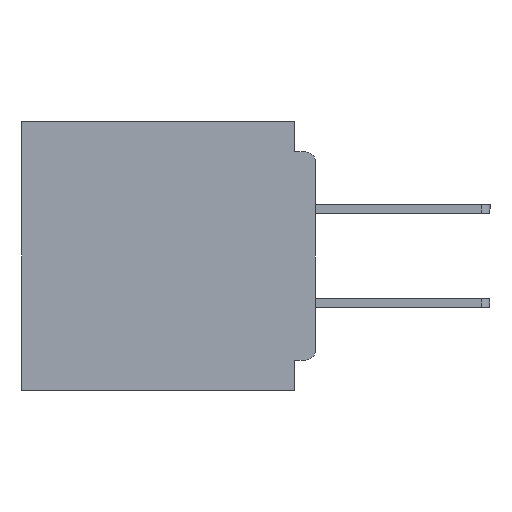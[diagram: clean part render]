
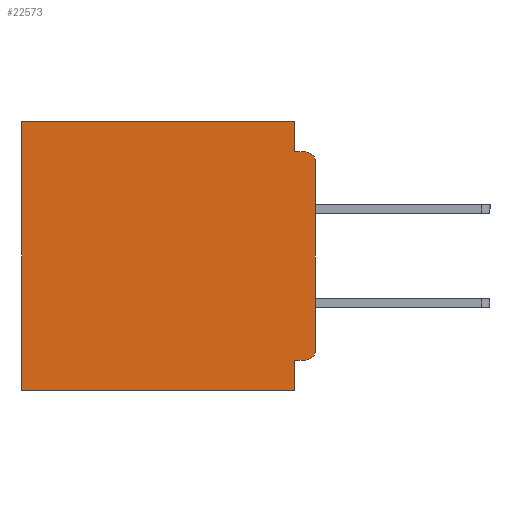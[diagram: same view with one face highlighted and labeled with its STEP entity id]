
A CAD part, left-side view. The second image highlights one B-rep face of the part: STEP entity #22573.
In plain terms, the highlighted planar face has unit normal (-1, 0, 0).
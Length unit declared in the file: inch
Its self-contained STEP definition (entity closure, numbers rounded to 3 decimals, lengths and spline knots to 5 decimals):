
#360 = CARTESIAN_POINT ( 'NONE',  ( 0.3, 0.031, -0.045 ) ) ;
#1058 = EDGE_CURVE ( 'NONE', #40323, #13940, #42511, .T. ) ;
#1134 = VECTOR ( 'NONE', #15272, 39.37008 ) ;
#2151 = AXIS2_PLACEMENT_3D ( 'NONE', #38801, #38703, #38646 ) ;
#2222 = LINE ( 'NONE', #35796, #1134 ) ;
#3002 = LINE ( 'NONE', #27524, #11056 ) ;
#3090 = PLANE ( 'NONE',  #3315 ) ;
#3315 = AXIS2_PLACEMENT_3D ( 'NONE', #33813, #13434, #37196 ) ;
#3655 = ORIENTED_EDGE ( 'NONE', *, *, #3857, .T. ) ;
#3857 = EDGE_CURVE ( 'NONE', #11465, #38300, #28055, .T. ) ;
#4116 = CARTESIAN_POINT ( 'NONE',  ( 0.3, 0., -0.34 ) ) ;
#4118 = ORIENTED_EDGE ( 'NONE', *, *, #21369, .F. ) ;
#5017 = EDGE_CURVE ( 'NONE', #40323, #13606, #28481, .T. ) ;
#5478 = ORIENTED_EDGE ( 'NONE', *, *, #30037, .T. ) ;
#6442 = VECTOR ( 'NONE', #20470, 39.37008 ) ;
#6855 = CARTESIAN_POINT ( 'NONE',  ( 0.3, 0.031, -0.355 ) ) ;
#6873 = ORIENTED_EDGE ( 'NONE', *, *, #43260, .F. ) ;
#7458 = DIRECTION ( 'NONE',  ( 0., 1., 0. ) ) ;
#8053 = VERTEX_POINT ( 'NONE', #24071 ) ;
#8957 = VECTOR ( 'NONE', #23183, 39.37008 ) ;
#9255 = ORIENTED_EDGE ( 'NONE', *, *, #5017, .T. ) ;
#10551 = DIRECTION ( 'NONE',  ( 0., 0., -1. ) ) ;
#10591 = EDGE_LOOP ( 'NONE', ( #35270, #9255, #6873, #4118, #3655, #15783, #39187, #33920, #41246, #5478 ) ) ;
#11056 = VECTOR ( 'NONE', #10551, 39.37008 ) ;
#11465 = VERTEX_POINT ( 'NONE', #25578 ) ;
#11623 = CARTESIAN_POINT ( 'NONE',  ( 0.3, 0., 0. ) ) ;
#12461 = DIRECTION ( 'NONE',  ( 0., 1., 0. ) ) ;
#13434 = DIRECTION ( 'NONE',  ( 1., 0., 0. ) ) ;
#13520 = VECTOR ( 'NONE', #39422, 39.37008 ) ;
#13606 = VERTEX_POINT ( 'NONE', #19066 ) ;
#13940 = VERTEX_POINT ( 'NONE', #4116 ) ;
#15272 = DIRECTION ( 'NONE',  ( 0., 0., -1. ) ) ;
#15783 = ORIENTED_EDGE ( 'NONE', *, *, #20322, .T. ) ;
#16253 = LINE ( 'NONE', #24460, #26403 ) ;
#16724 = CARTESIAN_POINT ( 'NONE',  ( 0.3, 0., -0.4 ) ) ;
#16883 = DIRECTION ( 'NONE',  ( 0., 1., 0. ) ) ;
#17685 = CARTESIAN_POINT ( 'NONE',  ( 0.3, 0.437, 0. ) ) ;
#18332 = CARTESIAN_POINT ( 'NONE',  ( 0.3, 0.015, -0.34 ) ) ;
#19066 = CARTESIAN_POINT ( 'NONE',  ( 0.3, 0.015, -0.045 ) ) ;
#19081 = CARTESIAN_POINT ( 'NONE',  ( 0.3, 0., -0.045 ) ) ;
#19359 = VERTEX_POINT ( 'NONE', #360 ) ;
#20322 = EDGE_CURVE ( 'NONE', #38300, #40238, #35038, .T. ) ;
#20384 = CIRCLE ( 'NONE', #27790, 0.015 ) ;
#20470 = DIRECTION ( 'NONE',  ( 0., 0., -1. ) ) ;
#21369 = EDGE_CURVE ( 'NONE', #11465, #19359, #3002, .T. ) ;
#21702 = CARTESIAN_POINT ( 'NONE',  ( 0.3, 0., -0.06 ) ) ;
#21775 = DIRECTION ( 'NONE',  ( 0., 0., -1. ) ) ;
#22573 = ADVANCED_FACE ( 'NONE', ( #36468 ), #3090, .F. ) ;
#22600 = EDGE_CURVE ( 'NONE', #24616, #40238, #16253, .T. ) ;
#22658 = CARTESIAN_POINT ( 'NONE',  ( 0.3, 0.031, -0.4 ) ) ;
#23183 = DIRECTION ( 'NONE',  ( 0., 0., -1. ) ) ;
#23650 = LINE ( 'NONE', #19081, #13520 ) ;
#23916 = EDGE_CURVE ( 'NONE', #32788, #24616, #2222, .T. ) ;
#24071 = CARTESIAN_POINT ( 'NONE',  ( 0.3, 0.015, -0.355 ) ) ;
#24460 = CARTESIAN_POINT ( 'NONE',  ( 0.3, 0., -0.4 ) ) ;
#24616 = VERTEX_POINT ( 'NONE', #22658 ) ;
#25578 = CARTESIAN_POINT ( 'NONE',  ( 0.3, 0.031, 0. ) ) ;
#25868 = VECTOR ( 'NONE', #12461, 39.37008 ) ;
#26403 = VECTOR ( 'NONE', #7458, 39.37008 ) ;
#27524 = CARTESIAN_POINT ( 'NONE',  ( 0.3, 0.031, 0. ) ) ;
#27790 = AXIS2_PLACEMENT_3D ( 'NONE', #18332, #42046, #21775 ) ;
#28055 = LINE ( 'NONE', #11623, #35974 ) ;
#28481 = CIRCLE ( 'NONE', #2151, 0.015 ) ;
#30037 = EDGE_CURVE ( 'NONE', #8053, #13940, #20384, .T. ) ;
#30041 = CARTESIAN_POINT ( 'NONE',  ( 0.3, 0.437, -0.4 ) ) ;
#32788 = VERTEX_POINT ( 'NONE', #6855 ) ;
#32862 = CARTESIAN_POINT ( 'NONE',  ( 0.3, 0., -0.355 ) ) ;
#33813 = CARTESIAN_POINT ( 'NONE',  ( 0.3, 0., -0.4 ) ) ;
#33920 = ORIENTED_EDGE ( 'NONE', *, *, #23916, .F. ) ;
#34905 = LINE ( 'NONE', #32862, #25868 ) ;
#34953 = CARTESIAN_POINT ( 'NONE',  ( 0.3, 0.437, -0.4 ) ) ;
#35038 = LINE ( 'NONE', #30041, #8957 ) ;
#35270 = ORIENTED_EDGE ( 'NONE', *, *, #1058, .F. ) ;
#35796 = CARTESIAN_POINT ( 'NONE',  ( 0.3, 0.031, -0.4 ) ) ;
#35974 = VECTOR ( 'NONE', #16883, 39.37008 ) ;
#36468 = FACE_OUTER_BOUND ( 'NONE', #10591, .T. ) ;
#37196 = DIRECTION ( 'NONE',  ( 0., 0., -1. ) ) ;
#38300 = VERTEX_POINT ( 'NONE', #17685 ) ;
#38590 = EDGE_CURVE ( 'NONE', #8053, #32788, #34905, .T. ) ;
#38646 = DIRECTION ( 'NONE',  ( 0., 0., -1. ) ) ;
#38703 = DIRECTION ( 'NONE',  ( -1., 0., 0. ) ) ;
#38801 = CARTESIAN_POINT ( 'NONE',  ( 0.3, 0.015, -0.06 ) ) ;
#39187 = ORIENTED_EDGE ( 'NONE', *, *, #22600, .F. ) ;
#39422 = DIRECTION ( 'NONE',  ( 0., -1., 0. ) ) ;
#40238 = VERTEX_POINT ( 'NONE', #34953 ) ;
#40323 = VERTEX_POINT ( 'NONE', #21702 ) ;
#41246 = ORIENTED_EDGE ( 'NONE', *, *, #38590, .F. ) ;
#42046 = DIRECTION ( 'NONE',  ( -1., 0., 0. ) ) ;
#42511 = LINE ( 'NONE', #16724, #6442 ) ;
#43260 = EDGE_CURVE ( 'NONE', #19359, #13606, #23650, .T. ) ;
